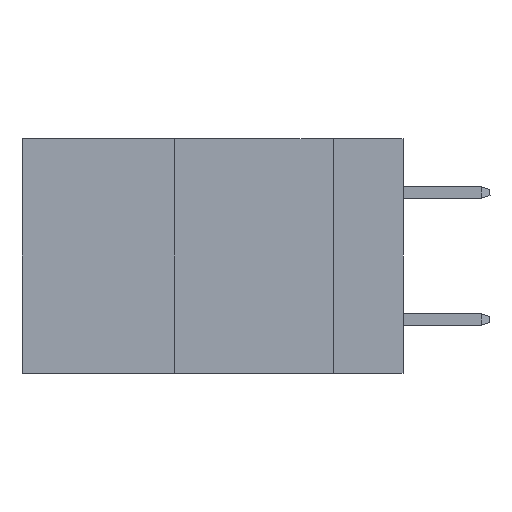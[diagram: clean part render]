
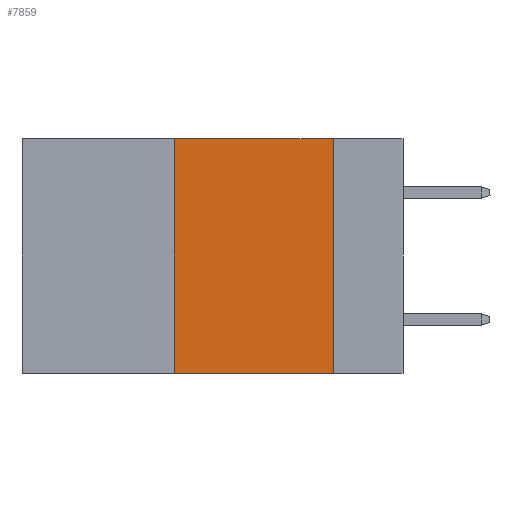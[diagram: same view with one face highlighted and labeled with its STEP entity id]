
A CAD part, left-side view. The second image highlights one B-rep face of the part: STEP entity #7859.
In plain terms, the highlighted planar face has unit normal (-1, 0, 0).
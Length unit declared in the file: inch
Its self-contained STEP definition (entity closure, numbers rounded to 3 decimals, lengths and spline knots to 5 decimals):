
#44 = CARTESIAN_POINT ( 'NONE',  ( 0., 0.6, 0. ) ) ;
#1248 = VERTEX_POINT ( 'NONE', #10846 ) ;
#1523 = DIRECTION ( 'NONE',  ( 0., 0., 1. ) ) ;
#1843 = VERTEX_POINT ( 'NONE', #11343 ) ;
#2903 = DIRECTION ( 'NONE',  ( 1., 0., 0. ) ) ;
#2989 = DIRECTION ( 'NONE',  ( 0., -1., 0. ) ) ;
#4105 = PLANE ( 'NONE',  #7016 ) ;
#4953 = ORIENTED_EDGE ( 'NONE', *, *, #11142, .F. ) ;
#5463 = LINE ( 'NONE', #11048, #16964 ) ;
#5670 = LINE ( 'NONE', #15555, #6158 ) ;
#5790 = CARTESIAN_POINT ( 'NONE',  ( 0., 0.11, -0.37 ) ) ;
#6158 = VECTOR ( 'NONE', #2989, 39.37008 ) ;
#7016 = AXIS2_PLACEMENT_3D ( 'NONE', #44, #2903, #8508 ) ;
#7448 = VERTEX_POINT ( 'NONE', #5790 ) ;
#7859 = ADVANCED_FACE ( 'NONE', ( #12621 ), #4105, .F. ) ;
#7914 = EDGE_CURVE ( 'NONE', #13056, #1248, #5670, .T. ) ;
#8319 = EDGE_CURVE ( 'NONE', #1843, #7448, #5463, .T. ) ;
#8508 = DIRECTION ( 'NONE',  ( 0., 0., -1. ) ) ;
#8555 = ORIENTED_EDGE ( 'NONE', *, *, #8319, .T. ) ;
#9773 = DIRECTION ( 'NONE',  ( 0., -1., 0. ) ) ;
#10359 = ORIENTED_EDGE ( 'NONE', *, *, #17034, .F. ) ;
#10498 = ORIENTED_EDGE ( 'NONE', *, *, #7914, .F. ) ;
#10635 = CARTESIAN_POINT ( 'NONE',  ( 0., 0.11, 0. ) ) ;
#10846 = CARTESIAN_POINT ( 'NONE',  ( 0., 0.11, 0. ) ) ;
#11048 = CARTESIAN_POINT ( 'NONE',  ( 0., 0.6, -0.37 ) ) ;
#11142 = EDGE_CURVE ( 'NONE', #1843, #13056, #12805, .T. ) ;
#11343 = CARTESIAN_POINT ( 'NONE',  ( 0., 0.36, -0.37 ) ) ;
#12173 = LINE ( 'NONE', #10635, #12210 ) ;
#12210 = VECTOR ( 'NONE', #14932, 39.37008 ) ;
#12480 = CARTESIAN_POINT ( 'NONE',  ( 0., 0.36, 0. ) ) ;
#12621 = FACE_OUTER_BOUND ( 'NONE', #14654, .T. ) ;
#12631 = CARTESIAN_POINT ( 'NONE',  ( 0., 0.36, 0. ) ) ;
#12805 = LINE ( 'NONE', #12631, #12877 ) ;
#12877 = VECTOR ( 'NONE', #1523, 39.37008 ) ;
#13056 = VERTEX_POINT ( 'NONE', #12480 ) ;
#14654 = EDGE_LOOP ( 'NONE', ( #10359, #10498, #4953, #8555 ) ) ;
#14932 = DIRECTION ( 'NONE',  ( 0., 0., -1. ) ) ;
#15555 = CARTESIAN_POINT ( 'NONE',  ( 0., 0.6, 0. ) ) ;
#16964 = VECTOR ( 'NONE', #9773, 39.37008 ) ;
#17034 = EDGE_CURVE ( 'NONE', #1248, #7448, #12173, .T. ) ;
